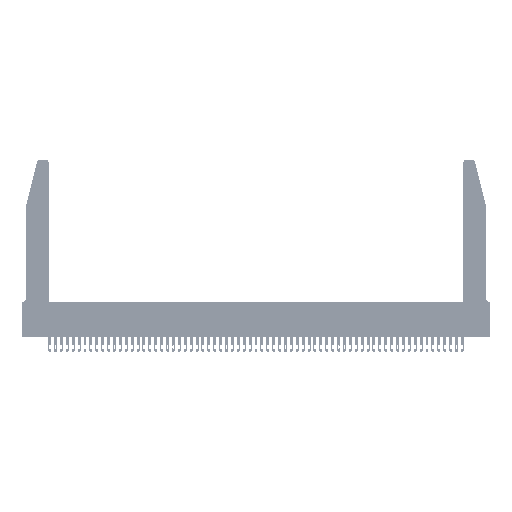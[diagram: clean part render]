
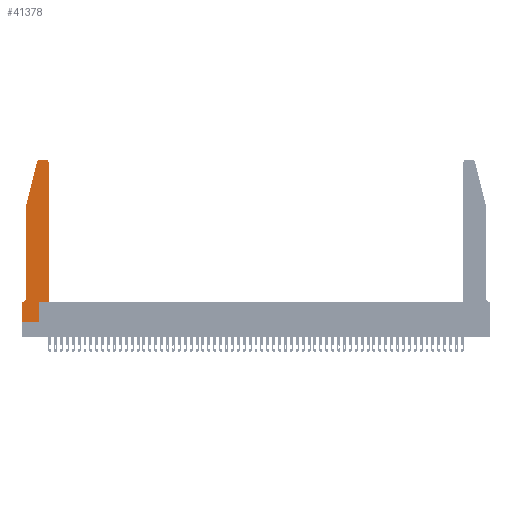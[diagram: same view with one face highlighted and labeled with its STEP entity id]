
A CAD part, top view. The second image highlights one B-rep face of the part: STEP entity #41378.
In plain terms, the highlighted planar face has unit normal (0, 0, 1).
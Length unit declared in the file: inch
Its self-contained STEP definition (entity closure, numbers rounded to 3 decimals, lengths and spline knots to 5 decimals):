
#965 = VECTOR ( 'NONE', #52005, 39.37008 ) ;
#2384 = ORIENTED_EDGE ( 'NONE', *, *, #3368, .T. ) ;
#2938 = DIRECTION ( 'NONE',  ( 1., 0., 0. ) ) ;
#3368 = EDGE_CURVE ( 'NONE', #42905, #18972, #6416, .T. ) ;
#3823 = CARTESIAN_POINT ( 'NONE',  ( 0.2865, 0.35, 0.37 ) ) ;
#3943 = CARTESIAN_POINT ( 'NONE',  ( 0.0755, 0.35, 0.37 ) ) ;
#4497 = ORIENTED_EDGE ( 'NONE', *, *, #34448, .T. ) ;
#4525 = CARTESIAN_POINT ( 'NONE',  ( 0.4505, 0.35, 0.37 ) ) ;
#4922 = VECTOR ( 'NONE', #18163, 39.37008 ) ;
#5543 = ORIENTED_EDGE ( 'NONE', *, *, #36850, .T. ) ;
#5673 = VERTEX_POINT ( 'NONE', #32443 ) ;
#5981 = ORIENTED_EDGE ( 'NONE', *, *, #46606, .T. ) ;
#6031 = LINE ( 'NONE', #8804, #34732 ) ;
#6416 = LINE ( 'NONE', #45950, #16662 ) ;
#7648 = CARTESIAN_POINT ( 'NONE',  ( 0.0755, 2., 0.37 ) ) ;
#7887 = ORIENTED_EDGE ( 'NONE', *, *, #30492, .T. ) ;
#8534 = DIRECTION ( 'NONE',  ( 0., 0., 1. ) ) ;
#8804 = CARTESIAN_POINT ( 'NONE',  ( 0., 0., 0.37 ) ) ;
#8897 = CARTESIAN_POINT ( 'NONE',  ( 0.284, 2.75, 0.37 ) ) ;
#10382 = VERTEX_POINT ( 'NONE', #17515 ) ;
#11421 = VERTEX_POINT ( 'NONE', #28267 ) ;
#12533 = LINE ( 'NONE', #7648, #22798 ) ;
#12558 = CARTESIAN_POINT ( 'NONE',  ( 0., 0.35, 0.37 ) ) ;
#13262 = ORIENTED_EDGE ( 'NONE', *, *, #37579, .T. ) ;
#13336 = DIRECTION ( 'NONE',  ( 0., 1., 0. ) ) ;
#15282 = ORIENTED_EDGE ( 'NONE', *, *, #46536, .T. ) ;
#15570 = EDGE_LOOP ( 'NONE', ( #2384, #5981, #17872, #5543, #15282, #13262, #7887, #39054, #43727, #27082, #4497, #25386 ) ) ;
#15712 = CARTESIAN_POINT ( 'NONE',  ( 0.4505, 0.35, 0.37 ) ) ;
#16522 = LINE ( 'NONE', #3943, #54773 ) ;
#16662 = VECTOR ( 'NONE', #23878, 39.37008 ) ;
#17515 = CARTESIAN_POINT ( 'NONE',  ( 0., 0.35, 0.37 ) ) ;
#17872 = ORIENTED_EDGE ( 'NONE', *, *, #27092, .T. ) ;
#17889 = DIRECTION ( 'NONE',  ( -1., 0., 0. ) ) ;
#18163 = DIRECTION ( 'NONE',  ( 0., 1., 0. ) ) ;
#18694 = AXIS2_PLACEMENT_3D ( 'NONE', #34814, #39046, #43593 ) ;
#18972 = VERTEX_POINT ( 'NONE', #8897 ) ;
#19432 = VERTEX_POINT ( 'NONE', #15712 ) ;
#19553 = LINE ( 'NONE', #38975, #4922 ) ;
#19787 = AXIS2_PLACEMENT_3D ( 'NONE', #47958, #56008, #26264 ) ;
#20601 = VECTOR ( 'NONE', #2938, 39.37008 ) ;
#21391 = CARTESIAN_POINT ( 'NONE',  ( 0.0755, 2., 0.37 ) ) ;
#22798 = VECTOR ( 'NONE', #42566, 39.37008 ) ;
#23127 = VERTEX_POINT ( 'NONE', #21391 ) ;
#23878 = DIRECTION ( 'NONE',  ( -1., 0., 0. ) ) ;
#24027 = LINE ( 'NONE', #33879, #20601 ) ;
#24583 = FACE_OUTER_BOUND ( 'NONE', #15570, .T. ) ;
#25293 = CARTESIAN_POINT ( 'NONE',  ( 0., 0., 0.37 ) ) ;
#25386 = ORIENTED_EDGE ( 'NONE', *, *, #41195, .T. ) ;
#25571 = DIRECTION ( 'NONE',  ( 1., 0., 0. ) ) ;
#26264 = DIRECTION ( 'NONE',  ( 1., 0., 0. ) ) ;
#26279 = CARTESIAN_POINT ( 'NONE',  ( 0.4505, 2.72, 0.37 ) ) ;
#27082 = ORIENTED_EDGE ( 'NONE', *, *, #38085, .T. ) ;
#27092 = EDGE_CURVE ( 'NONE', #11421, #23127, #30342, .T. ) ;
#27326 = VERTEX_POINT ( 'NONE', #48714 ) ;
#28267 = CARTESIAN_POINT ( 'NONE',  ( 0.25487, 2.72718, 0.37 ) ) ;
#28899 = VERTEX_POINT ( 'NONE', #26279 ) ;
#29929 = VERTEX_POINT ( 'NONE', #41233 ) ;
#30020 = VECTOR ( 'NONE', #51552, 39.37008 ) ;
#30342 = LINE ( 'NONE', #34638, #965 ) ;
#30492 = EDGE_CURVE ( 'NONE', #10382, #32152, #41607, .T. ) ;
#31499 = CARTESIAN_POINT ( 'NONE',  ( 0.4205, 2.75, 0.37 ) ) ;
#31846 = VECTOR ( 'NONE', #13336, 39.37008 ) ;
#32152 = VERTEX_POINT ( 'NONE', #42844 ) ;
#32443 = CARTESIAN_POINT ( 'NONE',  ( 0.2865, 0., 0.37 ) ) ;
#32672 = EDGE_CURVE ( 'NONE', #5673, #39035, #19553, .T. ) ;
#33160 = DIRECTION ( 'NONE',  ( 0., 0., 1. ) ) ;
#33879 = CARTESIAN_POINT ( 'NONE',  ( 0.4505, 0.35, 0.37 ) ) ;
#34448 = EDGE_CURVE ( 'NONE', #19432, #28899, #46168, .T. ) ;
#34493 = CIRCLE ( 'NONE', #18694, 0.07 ) ;
#34497 = PLANE ( 'NONE',  #40820 ) ;
#34638 = CARTESIAN_POINT ( 'NONE',  ( 0.0755, 2., 0.37 ) ) ;
#34732 = VECTOR ( 'NONE', #51924, 39.37008 ) ;
#34814 = CARTESIAN_POINT ( 'NONE',  ( 0.0055, 0.42, 0.37 ) ) ;
#36850 = EDGE_CURVE ( 'NONE', #23127, #29929, #12533, .T. ) ;
#37579 = EDGE_CURVE ( 'NONE', #27326, #10382, #16522, .T. ) ;
#38085 = EDGE_CURVE ( 'NONE', #39035, #19432, #24027, .T. ) ;
#38975 = CARTESIAN_POINT ( 'NONE',  ( 0.2865, 0.35, 0.37 ) ) ;
#39035 = VERTEX_POINT ( 'NONE', #3823 ) ;
#39046 = DIRECTION ( 'NONE',  ( 0., 0., -1. ) ) ;
#39054 = ORIENTED_EDGE ( 'NONE', *, *, #55298, .T. ) ;
#40820 = AXIS2_PLACEMENT_3D ( 'NONE', #12558, #8534, #25571 ) ;
#41195 = EDGE_CURVE ( 'NONE', #28899, #42905, #50470, .T. ) ;
#41198 = DIRECTION ( 'NONE',  ( 1., 0., 0. ) ) ;
#41233 = CARTESIAN_POINT ( 'NONE',  ( 0.0755, 0.42, 0.37 ) ) ;
#41378 = ADVANCED_FACE ( 'NONE', ( #24583 ), #34497, .T. ) ;
#41607 = LINE ( 'NONE', #25293, #30020 ) ;
#41757 = CARTESIAN_POINT ( 'NONE',  ( 0.4205, 2.72, 0.37 ) ) ;
#42566 = DIRECTION ( 'NONE',  ( 0., -1., 0. ) ) ;
#42844 = CARTESIAN_POINT ( 'NONE',  ( 0., 0., 0.37 ) ) ;
#42905 = VERTEX_POINT ( 'NONE', #31499 ) ;
#43593 = DIRECTION ( 'NONE',  ( -1., 0., 0. ) ) ;
#43727 = ORIENTED_EDGE ( 'NONE', *, *, #32672, .T. ) ;
#45950 = CARTESIAN_POINT ( 'NONE',  ( 0.2605, 2.75, 0.37 ) ) ;
#46168 = LINE ( 'NONE', #4525, #31846 ) ;
#46536 = EDGE_CURVE ( 'NONE', #29929, #27326, #34493, .T. ) ;
#46606 = EDGE_CURVE ( 'NONE', #18972, #11421, #53518, .T. ) ;
#47958 = CARTESIAN_POINT ( 'NONE',  ( 0.284, 2.72, 0.37 ) ) ;
#48714 = CARTESIAN_POINT ( 'NONE',  ( 0.0055, 0.35, 0.37 ) ) ;
#49591 = AXIS2_PLACEMENT_3D ( 'NONE', #41757, #33160, #41198 ) ;
#50470 = CIRCLE ( 'NONE', #49591, 0.03 ) ;
#51552 = DIRECTION ( 'NONE',  ( 0., -1., 0. ) ) ;
#51924 = DIRECTION ( 'NONE',  ( 1., 0., 0. ) ) ;
#52005 = DIRECTION ( 'NONE',  ( -0.239, -0.971, 0. ) ) ;
#53518 = CIRCLE ( 'NONE', #19787, 0.03 ) ;
#54773 = VECTOR ( 'NONE', #17889, 39.37008 ) ;
#55298 = EDGE_CURVE ( 'NONE', #32152, #5673, #6031, .T. ) ;
#56008 = DIRECTION ( 'NONE',  ( 0., 0., 1. ) ) ;
